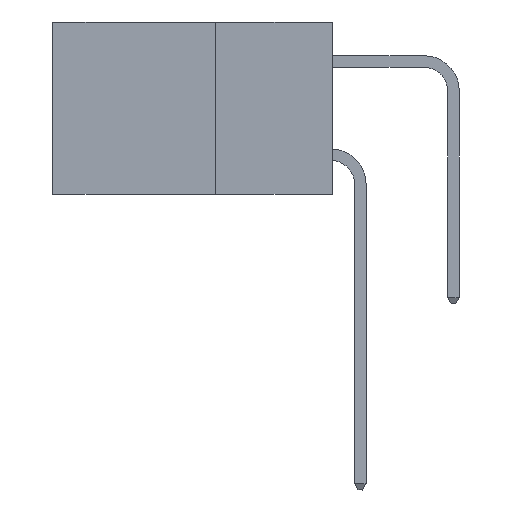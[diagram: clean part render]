
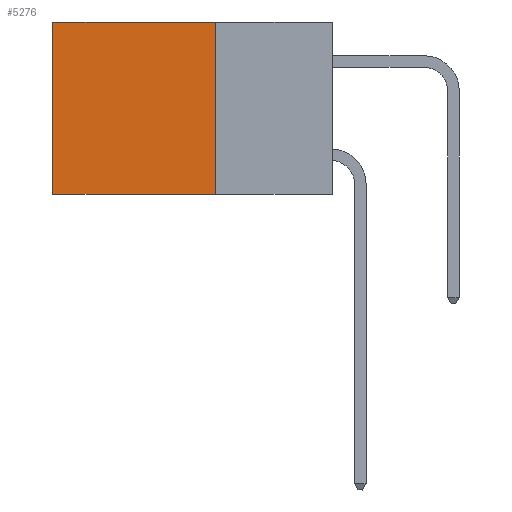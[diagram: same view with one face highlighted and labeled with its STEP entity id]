
A CAD part, left-side view. The second image highlights one B-rep face of the part: STEP entity #5276.
In plain terms, the highlighted planar face has unit normal (-1, 0, 0).
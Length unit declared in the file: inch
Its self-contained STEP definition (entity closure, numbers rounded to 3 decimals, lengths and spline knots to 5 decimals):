
#1781 = VECTOR ( 'NONE', #29352, 39.37008 ) ;
#2312 = LINE ( 'NONE', #19851, #20803 ) ;
#2343 = VECTOR ( 'NONE', #16929, 39.37008 ) ;
#4123 = LINE ( 'NONE', #25836, #21146 ) ;
#4544 = ORIENTED_EDGE ( 'NONE', *, *, #21950, .F. ) ;
#4669 = EDGE_LOOP ( 'NONE', ( #4681, #22762, #4544, #25426 ) ) ;
#4681 = ORIENTED_EDGE ( 'NONE', *, *, #18597, .T. ) ;
#5033 = DIRECTION ( 'NONE',  ( 0., 0., -1. ) ) ;
#5276 = ADVANCED_FACE ( 'NONE', ( #20620 ), #7380, .F. ) ;
#6688 = VERTEX_POINT ( 'NONE', #12363 ) ;
#7380 = PLANE ( 'NONE',  #21861 ) ;
#9211 = CARTESIAN_POINT ( 'NONE',  ( 0.298, 0.25, 0. ) ) ;
#9697 = DIRECTION ( 'NONE',  ( 1., 0., 0. ) ) ;
#10955 = CARTESIAN_POINT ( 'NONE',  ( 0.298, 0.25, 0. ) ) ;
#12259 = CARTESIAN_POINT ( 'NONE',  ( 0.298, 0.25, 0. ) ) ;
#12363 = CARTESIAN_POINT ( 'NONE',  ( 0.298, 0.25, -0.37 ) ) ;
#12956 = CARTESIAN_POINT ( 'NONE',  ( 0.298, 0.6, -0.37 ) ) ;
#13180 = EDGE_CURVE ( 'NONE', #6688, #14837, #2312, .T. ) ;
#13944 = VERTEX_POINT ( 'NONE', #18195 ) ;
#14837 = VERTEX_POINT ( 'NONE', #12956 ) ;
#15244 = DIRECTION ( 'NONE',  ( 0., 1., 0. ) ) ;
#16929 = DIRECTION ( 'NONE',  ( 0., 1., 0. ) ) ;
#17984 = EDGE_CURVE ( 'NONE', #21406, #13944, #26902, .T. ) ;
#18195 = CARTESIAN_POINT ( 'NONE',  ( 0.298, 0.6, 0. ) ) ;
#18597 = EDGE_CURVE ( 'NONE', #13944, #14837, #4123, .T. ) ;
#19851 = CARTESIAN_POINT ( 'NONE',  ( 0.298, 0.25, -0.37 ) ) ;
#20620 = FACE_OUTER_BOUND ( 'NONE', #4669, .T. ) ;
#20803 = VECTOR ( 'NONE', #15244, 39.37008 ) ;
#21146 = VECTOR ( 'NONE', #5033, 39.37008 ) ;
#21234 = CARTESIAN_POINT ( 'NONE',  ( 0.298, 0.25, 0. ) ) ;
#21406 = VERTEX_POINT ( 'NONE', #9211 ) ;
#21861 = AXIS2_PLACEMENT_3D ( 'NONE', #21234, #9697, #25833 ) ;
#21950 = EDGE_CURVE ( 'NONE', #21406, #6688, #26342, .T. ) ;
#22762 = ORIENTED_EDGE ( 'NONE', *, *, #13180, .F. ) ;
#25426 = ORIENTED_EDGE ( 'NONE', *, *, #17984, .T. ) ;
#25833 = DIRECTION ( 'NONE',  ( 0., 0., -1. ) ) ;
#25836 = CARTESIAN_POINT ( 'NONE',  ( 0.298, 0.6, 0. ) ) ;
#26342 = LINE ( 'NONE', #10955, #1781 ) ;
#26902 = LINE ( 'NONE', #12259, #2343 ) ;
#29352 = DIRECTION ( 'NONE',  ( 0., 0., -1. ) ) ;
